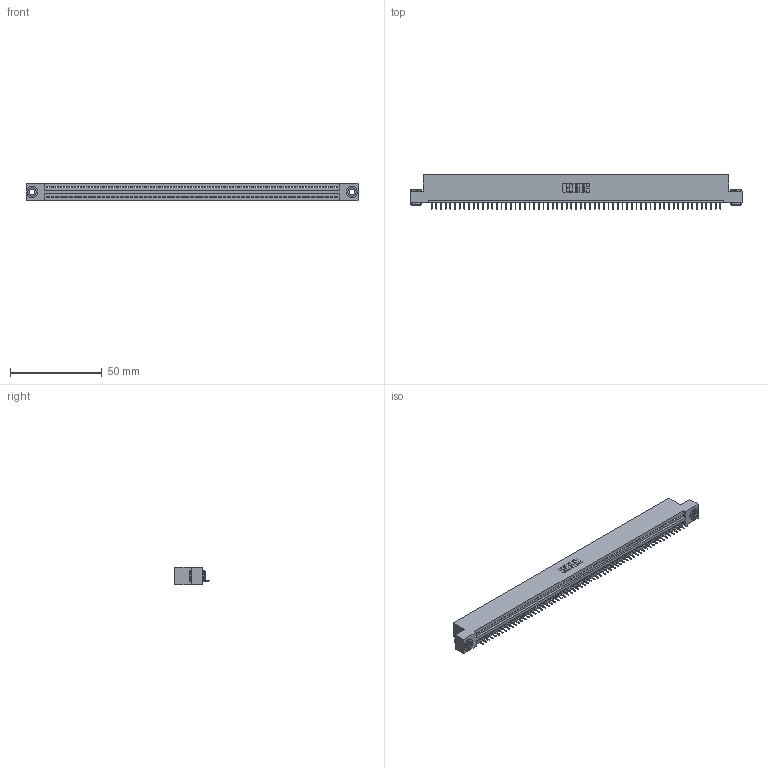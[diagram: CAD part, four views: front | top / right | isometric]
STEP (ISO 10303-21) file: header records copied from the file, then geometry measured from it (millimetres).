
FILE_DESCRIPTION (( 'STEP AP203' ), '1' );
FILE_NAME ('395-063-525-103.STEP', '2020-09-24T22:43:30', ( '' ), ( '' ), 'SwSTEP 2.0', 'SolidWorks 2020', '' );
FILE_SCHEMA (( 'CONFIG_CONTROL_DESIGN' ));
Length unit declared in the file: inch
Products named in the file (4): 345-250-002_345-250-002-102; 345-292-001_345-293-125; 395-063-525-103; 345 Part_Flush Mounting Lugs - 0.156 Dia-TH
Assembly tree (66 placements, depth 2):
  395-063-525-103
    345 Part_Flush Mounting Lugs - 0.156 Dia-TH
    345-292-001_345-293-125  x63
    345-250-002_345-250-002-102  x2
Bounding box: 181.23 x 18.72 x 9.4 mm (x, y, z)
Volume: 17147.5 mm3; surface area: 22429.6 mm2
Topology: 66 solids, 66 shells, 4070 faces, 11757 edges, 7582 vertices
Faces by surface type: plane 2988, cylinder 1074, cone 8
Entity records: 45312 total; most frequent: CARTESIAN_POINT 7824, ORIENTED_EDGE 7814, DIRECTION 6835, EDGE_CURVE 3907, VECTOR 3503, LINE 3503, VERTEX_POINT 2598, AXIS2_PLACEMENT_3D 1666
